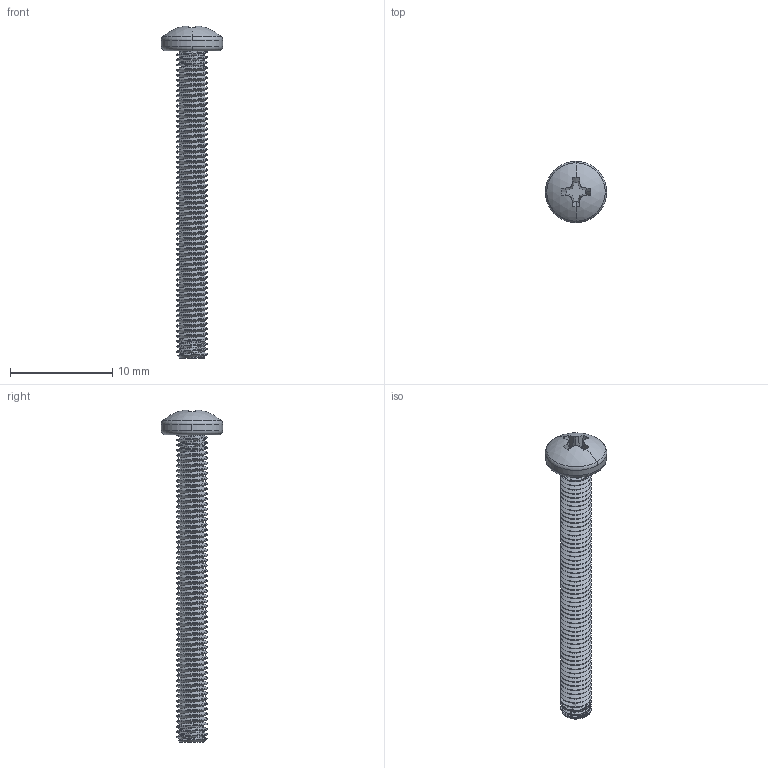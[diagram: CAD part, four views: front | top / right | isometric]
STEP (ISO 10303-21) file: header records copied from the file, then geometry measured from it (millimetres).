
FILE_DESCRIPTION (( 'STEP AP214' ), '1' );
FILE_NAME ('M3_30mm.step', '2015-06-12T16:04:05', ( '' ), ( '' ), 'SwSTEP 2.0', 'SolidWorks 2015', '' );
FILE_SCHEMA (( 'AUTOMOTIVE_DESIGN' ));
Length unit declared in the file: millimetre
Products named in the file (1): M3_30mm
Bounding box: 6 x 6 x 32.44 mm (x, y, z)
Volume: 217.2 mm3; surface area: 535 mm2
Topology: 1 solids, 1 shells, 340 faces, 1006 edges, 669 vertices
Faces by surface type: cylinder 303, plane 19, cone 9, torus 4, bspline 3, sphere 2
Entity records: 16051 total; most frequent: CARTESIAN_POINT 8716, ORIENTED_EDGE 2012, DIRECTION 1120, EDGE_CURVE 1006, VERTEX_POINT 669, AXIS2_PLACEMENT_3D 393, EDGE_LOOP 341, ADVANCED_FACE 340
